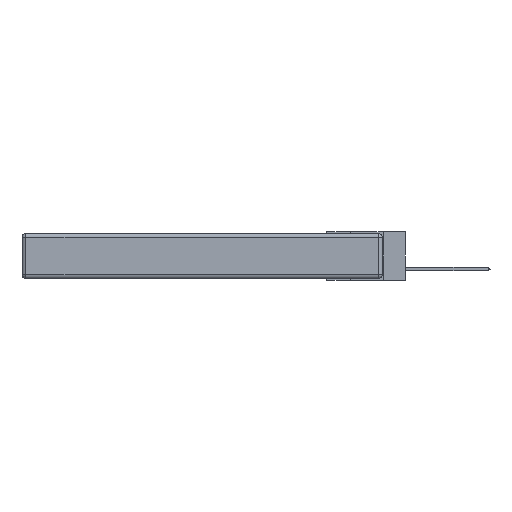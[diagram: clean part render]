
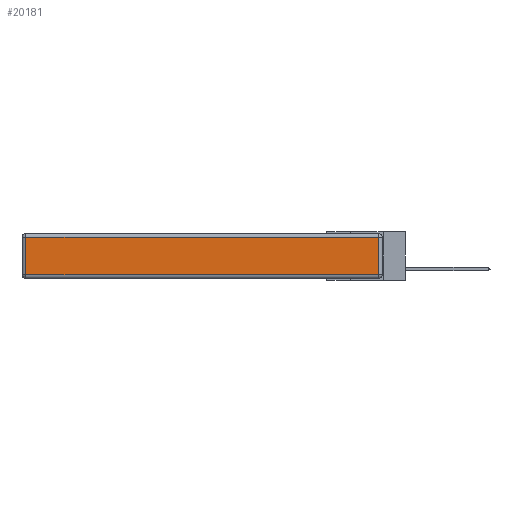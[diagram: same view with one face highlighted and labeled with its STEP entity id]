
A CAD part, left-side view. The second image highlights one B-rep face of the part: STEP entity #20181.
In plain terms, the highlighted planar face has unit normal (-1, 0, 0).
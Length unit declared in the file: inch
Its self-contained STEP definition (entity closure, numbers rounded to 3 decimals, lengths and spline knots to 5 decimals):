
#2118 = VERTEX_POINT ( 'NONE', #4960 ) ;
#2338 = LINE ( 'NONE', #3338, #17259 ) ;
#2346 = ORIENTED_EDGE ( 'NONE', *, *, #17066, .T. ) ;
#3247 = VECTOR ( 'NONE', #18432, 39.37008 ) ;
#3338 = CARTESIAN_POINT ( 'NONE',  ( 0., 0., -0.313 ) ) ;
#4629 = PLANE ( 'NONE',  #5491 ) ;
#4740 = VERTEX_POINT ( 'NONE', #11487 ) ;
#4960 = CARTESIAN_POINT ( 'NONE',  ( 0., 2.72, -0.03 ) ) ;
#4986 = ORIENTED_EDGE ( 'NONE', *, *, #15612, .T. ) ;
#5491 = AXIS2_PLACEMENT_3D ( 'NONE', #12843, #15927, #15860 ) ;
#5790 = LINE ( 'NONE', #16451, #16253 ) ;
#6914 = DIRECTION ( 'NONE',  ( 0., 1., 0. ) ) ;
#7841 = VECTOR ( 'NONE', #9020, 39.37008 ) ;
#7940 = FACE_OUTER_BOUND ( 'NONE', #18083, .T. ) ;
#8181 = VERTEX_POINT ( 'NONE', #9518 ) ;
#9020 = DIRECTION ( 'NONE',  ( 0., 0., -1. ) ) ;
#9034 = ORIENTED_EDGE ( 'NONE', *, *, #10218, .T. ) ;
#9425 = DIRECTION ( 'NONE',  ( 0., -1., 0. ) ) ;
#9518 = CARTESIAN_POINT ( 'NONE',  ( 0., 0.03, -0.313 ) ) ;
#10041 = CARTESIAN_POINT ( 'NONE',  ( 0., 0.03, -0.343 ) ) ;
#10218 = EDGE_CURVE ( 'NONE', #2118, #20493, #16326, .T. ) ;
#11487 = CARTESIAN_POINT ( 'NONE',  ( 0., 0.03, -0.03 ) ) ;
#12843 = CARTESIAN_POINT ( 'NONE',  ( 0., 0., -0.343 ) ) ;
#14480 = ORIENTED_EDGE ( 'NONE', *, *, #14961, .T. ) ;
#14961 = EDGE_CURVE ( 'NONE', #20493, #8181, #2338, .T. ) ;
#15396 = CARTESIAN_POINT ( 'NONE',  ( 0., 2.72, -0.343 ) ) ;
#15612 = EDGE_CURVE ( 'NONE', #4740, #2118, #5790, .T. ) ;
#15860 = DIRECTION ( 'NONE',  ( 0., 0., 1. ) ) ;
#15927 = DIRECTION ( 'NONE',  ( -1., 0., 0. ) ) ;
#16253 = VECTOR ( 'NONE', #6914, 39.37008 ) ;
#16326 = LINE ( 'NONE', #15396, #7841 ) ;
#16451 = CARTESIAN_POINT ( 'NONE',  ( 0., 2.75, -0.03 ) ) ;
#17066 = EDGE_CURVE ( 'NONE', #8181, #4740, #19153, .T. ) ;
#17259 = VECTOR ( 'NONE', #9425, 39.37008 ) ;
#18083 = EDGE_LOOP ( 'NONE', ( #14480, #2346, #4986, #9034 ) ) ;
#18432 = DIRECTION ( 'NONE',  ( 0., 0., 1. ) ) ;
#19153 = LINE ( 'NONE', #10041, #3247 ) ;
#20128 = CARTESIAN_POINT ( 'NONE',  ( 0., 2.72, -0.313 ) ) ;
#20181 = ADVANCED_FACE ( 'NONE', ( #7940 ), #4629, .T. ) ;
#20493 = VERTEX_POINT ( 'NONE', #20128 ) ;
